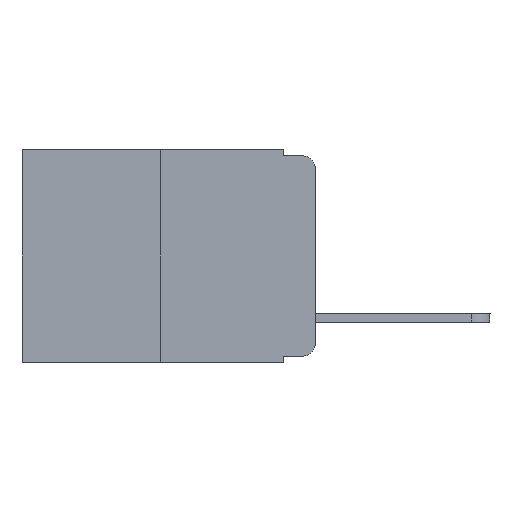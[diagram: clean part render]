
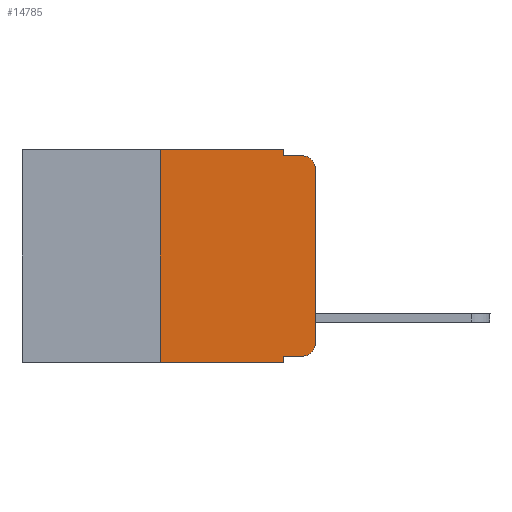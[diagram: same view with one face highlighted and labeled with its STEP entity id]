
A CAD part, left-side view. The second image highlights one B-rep face of the part: STEP entity #14785.
In plain terms, the highlighted planar face has unit normal (-1, 0, 0).
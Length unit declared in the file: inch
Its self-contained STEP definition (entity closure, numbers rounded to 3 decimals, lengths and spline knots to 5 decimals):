
#71 = DIRECTION ( 'NONE',  ( 0., 0., 1. ) ) ;
#195 = DIRECTION ( 'NONE',  ( 0., -1., 0. ) ) ;
#270 = EDGE_CURVE ( 'NONE', #16877, #13035, #844, .T. ) ;
#282 = VERTEX_POINT ( 'NONE', #2197 ) ;
#286 = AXIS2_PLACEMENT_3D ( 'NONE', #5966, #10006, #11411 ) ;
#326 = LINE ( 'NONE', #1470, #6834 ) ;
#390 = CARTESIAN_POINT ( 'NONE',  ( 0., 0., -0.03 ) ) ;
#392 = CARTESIAN_POINT ( 'NONE',  ( 0., 0.25, 0. ) ) ;
#688 = PLANE ( 'NONE',  #14128 ) ;
#731 = CARTESIAN_POINT ( 'NONE',  ( 0., 0.473, -0.343 ) ) ;
#844 = CIRCLE ( 'NONE', #286, 0.02 ) ;
#932 = LINE ( 'NONE', #2507, #11032 ) ;
#951 = LINE ( 'NONE', #2274, #9841 ) ;
#1162 = CARTESIAN_POINT ( 'NONE',  ( 0., 0.02, -0.313 ) ) ;
#1315 = EDGE_CURVE ( 'NONE', #282, #13321, #16327, .T. ) ;
#1470 = CARTESIAN_POINT ( 'NONE',  ( 0., 0.25, 0. ) ) ;
#1827 = CARTESIAN_POINT ( 'NONE',  ( 0., 0.051, 0. ) ) ;
#1886 = VECTOR ( 'NONE', #5189, 39.37008 ) ;
#2012 = DIRECTION ( 'NONE',  ( 1., 0., 0. ) ) ;
#2102 = EDGE_CURVE ( 'NONE', #13413, #10938, #14570, .T. ) ;
#2197 = CARTESIAN_POINT ( 'NONE',  ( 0., 0.051, 0. ) ) ;
#2213 = CARTESIAN_POINT ( 'NONE',  ( 0., 0.02, -0.01 ) ) ;
#2274 = CARTESIAN_POINT ( 'NONE',  ( 0., 0.051, -0.01 ) ) ;
#2507 = CARTESIAN_POINT ( 'NONE',  ( 0., 0.473, 0. ) ) ;
#2647 = LINE ( 'NONE', #17145, #1886 ) ;
#3320 = CARTESIAN_POINT ( 'NONE',  ( 0., 0.473, 0. ) ) ;
#3623 = VECTOR ( 'NONE', #12857, 39.37008 ) ;
#3856 = ORIENTED_EDGE ( 'NONE', *, *, #270, .T. ) ;
#3911 = AXIS2_PLACEMENT_3D ( 'NONE', #1162, #6681, #14602 ) ;
#3926 = VERTEX_POINT ( 'NONE', #16421 ) ;
#4054 = LINE ( 'NONE', #14843, #16176 ) ;
#4117 = ORIENTED_EDGE ( 'NONE', *, *, #1315, .F. ) ;
#4818 = DIRECTION ( 'NONE',  ( 0., 0., -1. ) ) ;
#4897 = EDGE_CURVE ( 'NONE', #15577, #8809, #8719, .T. ) ;
#5189 = DIRECTION ( 'NONE',  ( 0., 0., 1. ) ) ;
#5966 = CARTESIAN_POINT ( 'NONE',  ( 0., 0.02, -0.03 ) ) ;
#6290 = ORIENTED_EDGE ( 'NONE', *, *, #2102, .T. ) ;
#6544 = EDGE_CURVE ( 'NONE', #3926, #13413, #8261, .T. ) ;
#6681 = DIRECTION ( 'NONE',  ( -1., 0., 0. ) ) ;
#6834 = VECTOR ( 'NONE', #71, 39.37008 ) ;
#7152 = ORIENTED_EDGE ( 'NONE', *, *, #11450, .F. ) ;
#7207 = EDGE_CURVE ( 'NONE', #13321, #13035, #951, .T. ) ;
#8261 = LINE ( 'NONE', #11076, #12363 ) ;
#8719 = LINE ( 'NONE', #731, #3623 ) ;
#8809 = VERTEX_POINT ( 'NONE', #12197 ) ;
#9030 = EDGE_CURVE ( 'NONE', #11199, #282, #932, .T. ) ;
#9841 = VECTOR ( 'NONE', #10436, 39.37008 ) ;
#10006 = DIRECTION ( 'NONE',  ( -1., 0., 0. ) ) ;
#10017 = ORIENTED_EDGE ( 'NONE', *, *, #9030, .F. ) ;
#10172 = FACE_OUTER_BOUND ( 'NONE', #14074, .T. ) ;
#10233 = ORIENTED_EDGE ( 'NONE', *, *, #4897, .T. ) ;
#10436 = DIRECTION ( 'NONE',  ( 0., -1., 0. ) ) ;
#10931 = CARTESIAN_POINT ( 'NONE',  ( 0., 0.25, -0.343 ) ) ;
#10938 = VERTEX_POINT ( 'NONE', #13131 ) ;
#11032 = VECTOR ( 'NONE', #14544, 39.37008 ) ;
#11069 = ORIENTED_EDGE ( 'NONE', *, *, #15071, .F. ) ;
#11076 = CARTESIAN_POINT ( 'NONE',  ( 0., 0.051, -0.333 ) ) ;
#11199 = VERTEX_POINT ( 'NONE', #392 ) ;
#11246 = VECTOR ( 'NONE', #12463, 39.37008 ) ;
#11411 = DIRECTION ( 'NONE',  ( 0., 0., -1. ) ) ;
#11450 = EDGE_CURVE ( 'NONE', #3926, #8809, #4054, .T. ) ;
#11526 = ORIENTED_EDGE ( 'NONE', *, *, #13090, .T. ) ;
#11930 = CARTESIAN_POINT ( 'NONE',  ( 0., 0.02, -0.333 ) ) ;
#12197 = CARTESIAN_POINT ( 'NONE',  ( 0., 0.051, -0.343 ) ) ;
#12363 = VECTOR ( 'NONE', #195, 39.37008 ) ;
#12463 = DIRECTION ( 'NONE',  ( 0., 0., -1. ) ) ;
#12474 = CARTESIAN_POINT ( 'NONE',  ( 0., 0.051, -0.01 ) ) ;
#12857 = DIRECTION ( 'NONE',  ( 0., -1., 0. ) ) ;
#13035 = VERTEX_POINT ( 'NONE', #2213 ) ;
#13090 = EDGE_CURVE ( 'NONE', #10938, #16877, #2647, .T. ) ;
#13099 = ORIENTED_EDGE ( 'NONE', *, *, #6544, .T. ) ;
#13131 = CARTESIAN_POINT ( 'NONE',  ( 0., 0., -0.313 ) ) ;
#13321 = VERTEX_POINT ( 'NONE', #12474 ) ;
#13413 = VERTEX_POINT ( 'NONE', #11930 ) ;
#13624 = DIRECTION ( 'NONE',  ( 0., 0., -1. ) ) ;
#14074 = EDGE_LOOP ( 'NONE', ( #11526, #3856, #14747, #4117, #10017, #11069, #10233, #7152, #13099, #6290 ) ) ;
#14128 = AXIS2_PLACEMENT_3D ( 'NONE', #3320, #2012, #4818 ) ;
#14544 = DIRECTION ( 'NONE',  ( 0., -1., 0. ) ) ;
#14570 = CIRCLE ( 'NONE', #3911, 0.02 ) ;
#14602 = DIRECTION ( 'NONE',  ( 0., 0., -1. ) ) ;
#14747 = ORIENTED_EDGE ( 'NONE', *, *, #7207, .F. ) ;
#14785 = ADVANCED_FACE ( 'NONE', ( #10172 ), #688, .F. ) ;
#14843 = CARTESIAN_POINT ( 'NONE',  ( 0., 0.051, 0. ) ) ;
#15071 = EDGE_CURVE ( 'NONE', #15577, #11199, #326, .T. ) ;
#15577 = VERTEX_POINT ( 'NONE', #10931 ) ;
#16176 = VECTOR ( 'NONE', #13624, 39.37008 ) ;
#16327 = LINE ( 'NONE', #1827, #11246 ) ;
#16421 = CARTESIAN_POINT ( 'NONE',  ( 0., 0.051, -0.333 ) ) ;
#16877 = VERTEX_POINT ( 'NONE', #390 ) ;
#17145 = CARTESIAN_POINT ( 'NONE',  ( 0., 0., 0. ) ) ;
